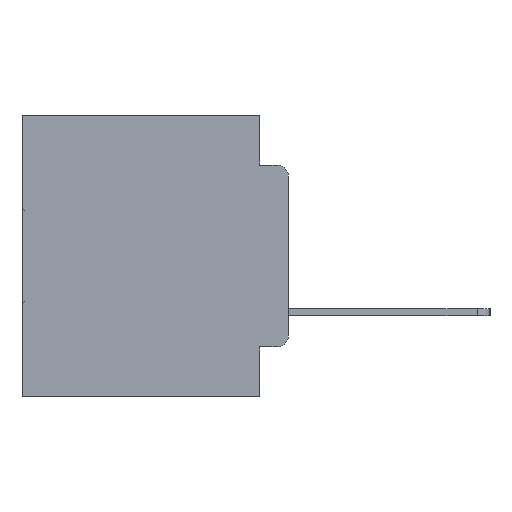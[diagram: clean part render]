
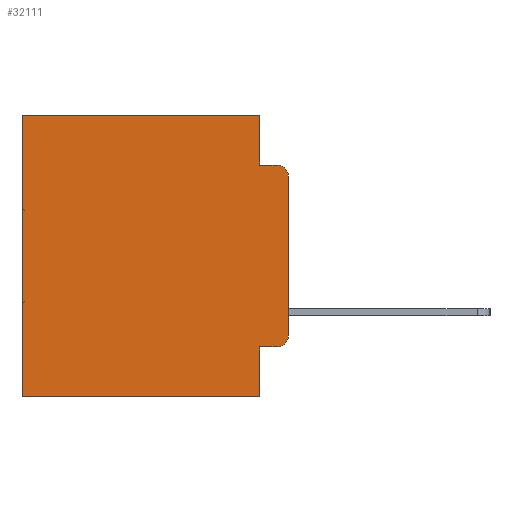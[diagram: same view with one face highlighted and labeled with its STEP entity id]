
A CAD part, left-side view. The second image highlights one B-rep face of the part: STEP entity #32111.
In plain terms, the highlighted planar face has unit normal (-1, 0, 0).
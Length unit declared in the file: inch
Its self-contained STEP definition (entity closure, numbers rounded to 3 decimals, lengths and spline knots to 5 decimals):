
#603 = EDGE_CURVE ( 'NONE', #26144, #3704, #26393, .T. ) ;
#676 = DIRECTION ( 'NONE',  ( 0., -1., 0. ) ) ;
#1331 = EDGE_CURVE ( 'NONE', #26144, #9500, #21251, .T. ) ;
#1416 = CARTESIAN_POINT ( 'NONE',  ( 0.298, 0., 0. ) ) ;
#1534 = EDGE_CURVE ( 'NONE', #9500, #3094, #25886, .T. ) ;
#2351 = EDGE_CURVE ( 'NONE', #5142, #3094, #5503, .T. ) ;
#3094 = VERTEX_POINT ( 'NONE', #15879 ) ;
#3494 = ORIENTED_EDGE ( 'NONE', *, *, #23201, .F. ) ;
#3602 = ORIENTED_EDGE ( 'NONE', *, *, #9982, .T. ) ;
#3704 = VERTEX_POINT ( 'NONE', #9173 ) ;
#4024 = CARTESIAN_POINT ( 'NONE',  ( 0.298, 0.051, -0.0885 ) ) ;
#4042 = DIRECTION ( 'NONE',  ( 0., 0., -1. ) ) ;
#4082 = CIRCLE ( 'NONE', #20065, 0.02 ) ;
#4641 = CARTESIAN_POINT ( 'NONE',  ( 0.298, 0., -0.5 ) ) ;
#5142 = VERTEX_POINT ( 'NONE', #7574 ) ;
#5503 = LINE ( 'NONE', #31959, #12238 ) ;
#5973 = VECTOR ( 'NONE', #17441, 39.37008 ) ;
#6277 = CARTESIAN_POINT ( 'NONE',  ( 0.298, 0.02, -0.1085 ) ) ;
#6365 = ORIENTED_EDGE ( 'NONE', *, *, #2351, .T. ) ;
#6460 = VECTOR ( 'NONE', #15349, 39.37008 ) ;
#7198 = ORIENTED_EDGE ( 'NONE', *, *, #16169, .F. ) ;
#7560 = VERTEX_POINT ( 'NONE', #10145 ) ;
#7574 = CARTESIAN_POINT ( 'NONE',  ( 0.298, 0.473, 0. ) ) ;
#8397 = CARTESIAN_POINT ( 'NONE',  ( 0.298, 0.051, -0.0885 ) ) ;
#8435 = CARTESIAN_POINT ( 'NONE',  ( 0.298, 0.02, -0.3915 ) ) ;
#8448 = CARTESIAN_POINT ( 'NONE',  ( 0.298, 0.02, -0.0885 ) ) ;
#8779 = ORIENTED_EDGE ( 'NONE', *, *, #1534, .F. ) ;
#8811 = DIRECTION ( 'NONE',  ( 0., 0., -1. ) ) ;
#8816 = CARTESIAN_POINT ( 'NONE',  ( 0.298, 0.051, -0.4115 ) ) ;
#9160 = ORIENTED_EDGE ( 'NONE', *, *, #1331, .F. ) ;
#9173 = CARTESIAN_POINT ( 'NONE',  ( 0.298, 0.02, -0.4115 ) ) ;
#9205 = ORIENTED_EDGE ( 'NONE', *, *, #13006, .T. ) ;
#9389 = VERTEX_POINT ( 'NONE', #4024 ) ;
#9500 = VERTEX_POINT ( 'NONE', #19563 ) ;
#9982 = EDGE_CURVE ( 'NONE', #24519, #5142, #27912, .T. ) ;
#10145 = CARTESIAN_POINT ( 'NONE',  ( 0.298, 0., -0.1085 ) ) ;
#10351 = ORIENTED_EDGE ( 'NONE', *, *, #603, .T. ) ;
#10397 = ORIENTED_EDGE ( 'NONE', *, *, #31963, .T. ) ;
#10982 = DIRECTION ( 'NONE',  ( 0., 0., -1. ) ) ;
#12238 = VECTOR ( 'NONE', #14740, 39.37008 ) ;
#12258 = EDGE_CURVE ( 'NONE', #7560, #28014, #12733, .T. ) ;
#12733 = LINE ( 'NONE', #13602, #31660 ) ;
#13006 = EDGE_CURVE ( 'NONE', #7560, #19881, #23920, .T. ) ;
#13602 = CARTESIAN_POINT ( 'NONE',  ( 0.298, 0., 0. ) ) ;
#13718 = DIRECTION ( 'NONE',  ( 0., 0., -1. ) ) ;
#14343 = CARTESIAN_POINT ( 'NONE',  ( 0.298, 0.051, 0. ) ) ;
#14595 = VECTOR ( 'NONE', #676, 39.37008 ) ;
#14740 = DIRECTION ( 'NONE',  ( 0., 0., -1. ) ) ;
#14743 = CARTESIAN_POINT ( 'NONE',  ( 0.298, 0.051, 0. ) ) ;
#15349 = DIRECTION ( 'NONE',  ( 0., -1., 0. ) ) ;
#15526 = VECTOR ( 'NONE', #21902, 39.37008 ) ;
#15879 = CARTESIAN_POINT ( 'NONE',  ( 0.298, 0.473, -0.5 ) ) ;
#16169 = EDGE_CURVE ( 'NONE', #24519, #9389, #25431, .T. ) ;
#16193 = AXIS2_PLACEMENT_3D ( 'NONE', #1416, #19149, #4042 ) ;
#16313 = VECTOR ( 'NONE', #30040, 39.37008 ) ;
#16719 = PLANE ( 'NONE',  #16193 ) ;
#17441 = DIRECTION ( 'NONE',  ( 0., 1., 0. ) ) ;
#19149 = DIRECTION ( 'NONE',  ( 1., 0., 0. ) ) ;
#19269 = DIRECTION ( 'NONE',  ( 0., 0., -1. ) ) ;
#19563 = CARTESIAN_POINT ( 'NONE',  ( 0.298, 0.051, -0.5 ) ) ;
#19881 = VERTEX_POINT ( 'NONE', #8448 ) ;
#20065 = AXIS2_PLACEMENT_3D ( 'NONE', #8435, #25868, #10982 ) ;
#20084 = CARTESIAN_POINT ( 'NONE',  ( 0.298, 0.051, -0.4115 ) ) ;
#20376 = VECTOR ( 'NONE', #19269, 39.37008 ) ;
#21251 = LINE ( 'NONE', #14743, #15526 ) ;
#21902 = DIRECTION ( 'NONE',  ( 0., 0., -1. ) ) ;
#23201 = EDGE_CURVE ( 'NONE', #9389, #19881, #29278, .T. ) ;
#23777 = DIRECTION ( 'NONE',  ( -1., 0., 0. ) ) ;
#23920 = CIRCLE ( 'NONE', #31727, 0.02 ) ;
#24519 = VERTEX_POINT ( 'NONE', #30205 ) ;
#25431 = LINE ( 'NONE', #14343, #20376 ) ;
#25868 = DIRECTION ( 'NONE',  ( -1., 0., 0. ) ) ;
#25886 = LINE ( 'NONE', #4641, #5973 ) ;
#26144 = VERTEX_POINT ( 'NONE', #8816 ) ;
#26393 = LINE ( 'NONE', #20084, #6460 ) ;
#26715 = ORIENTED_EDGE ( 'NONE', *, *, #12258, .F. ) ;
#27236 = CARTESIAN_POINT ( 'NONE',  ( 0.298, 0., -0.3915 ) ) ;
#27571 = CARTESIAN_POINT ( 'NONE',  ( 0.298, 0., 0. ) ) ;
#27912 = LINE ( 'NONE', #27571, #16313 ) ;
#28014 = VERTEX_POINT ( 'NONE', #27236 ) ;
#29278 = LINE ( 'NONE', #8397, #14595 ) ;
#30040 = DIRECTION ( 'NONE',  ( 0., 1., 0. ) ) ;
#30205 = CARTESIAN_POINT ( 'NONE',  ( 0.298, 0.051, 0. ) ) ;
#30373 = EDGE_LOOP ( 'NONE', ( #26715, #9205, #3494, #7198, #3602, #6365, #8779, #9160, #10351, #10397 ) ) ;
#31660 = VECTOR ( 'NONE', #13718, 39.37008 ) ;
#31727 = AXIS2_PLACEMENT_3D ( 'NONE', #6277, #23777, #8811 ) ;
#31959 = CARTESIAN_POINT ( 'NONE',  ( 0.298, 0.473, 0. ) ) ;
#31963 = EDGE_CURVE ( 'NONE', #3704, #28014, #4082, .T. ) ;
#32111 = ADVANCED_FACE ( 'NONE', ( #32544 ), #16719, .F. ) ;
#32544 = FACE_OUTER_BOUND ( 'NONE', #30373, .T. ) ;
